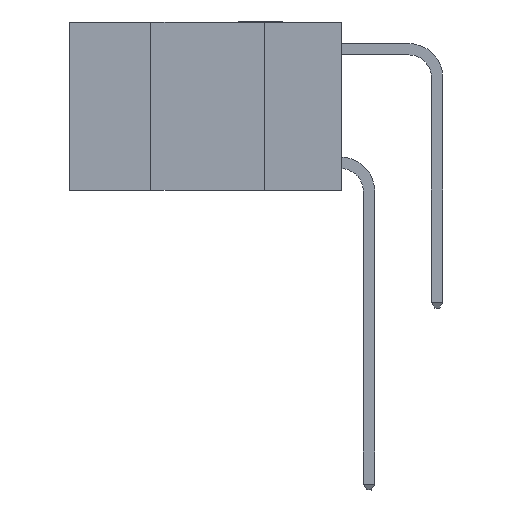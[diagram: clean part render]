
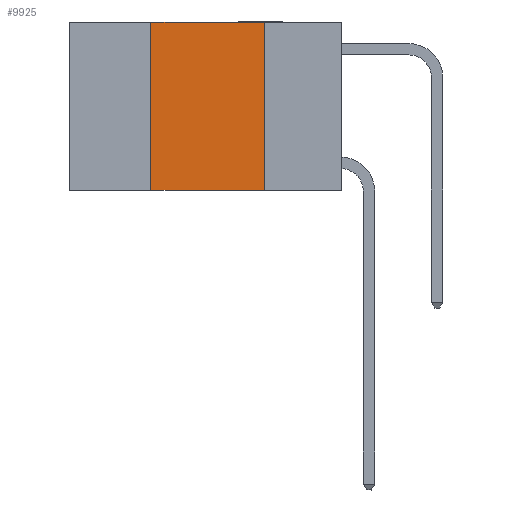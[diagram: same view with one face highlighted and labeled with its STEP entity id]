
A CAD part, left-side view. The second image highlights one B-rep face of the part: STEP entity #9925.
In plain terms, the highlighted planar face has unit normal (-1, 0, 0).
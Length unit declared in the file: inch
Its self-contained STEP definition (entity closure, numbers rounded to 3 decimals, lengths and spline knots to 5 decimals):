
#55 = EDGE_LOOP ( 'NONE', ( #5130, #11378, #8687, #7718 ) ) ;
#657 = AXIS2_PLACEMENT_3D ( 'NONE', #778, #5902, #2843 ) ;
#673 = EDGE_CURVE ( 'NONE', #7932, #5850, #7061, .T. ) ;
#778 = CARTESIAN_POINT ( 'NONE',  ( 0., 0.6, 0. ) ) ;
#857 = DIRECTION ( 'NONE',  ( 0., 0., -1. ) ) ;
#1507 = CARTESIAN_POINT ( 'NONE',  ( 0., 0.42, -0.37 ) ) ;
#1593 = EDGE_CURVE ( 'NONE', #3662, #11846, #10173, .T. ) ;
#2390 = LINE ( 'NONE', #8890, #10620 ) ;
#2830 = EDGE_CURVE ( 'NONE', #11846, #7932, #9328, .T. ) ;
#2843 = DIRECTION ( 'NONE',  ( 0., 0., -1. ) ) ;
#3420 = VECTOR ( 'NONE', #6215, 39.37008 ) ;
#3501 = CARTESIAN_POINT ( 'NONE',  ( 0., 0.17, -0.37 ) ) ;
#3662 = VERTEX_POINT ( 'NONE', #1507 ) ;
#4365 = CARTESIAN_POINT ( 'NONE',  ( 0., 0.6, 0. ) ) ;
#4550 = CARTESIAN_POINT ( 'NONE',  ( 0., 0.42, 0. ) ) ;
#5130 = ORIENTED_EDGE ( 'NONE', *, *, #673, .F. ) ;
#5850 = VERTEX_POINT ( 'NONE', #3501 ) ;
#5902 = DIRECTION ( 'NONE',  ( 1., 0., 0. ) ) ;
#6038 = DIRECTION ( 'NONE',  ( 0., 0., 1. ) ) ;
#6215 = DIRECTION ( 'NONE',  ( 0., -1., 0. ) ) ;
#7061 = LINE ( 'NONE', #8908, #9353 ) ;
#7544 = FACE_OUTER_BOUND ( 'NONE', #55, .T. ) ;
#7718 = ORIENTED_EDGE ( 'NONE', *, *, #11146, .T. ) ;
#7932 = VERTEX_POINT ( 'NONE', #11216 ) ;
#8687 = ORIENTED_EDGE ( 'NONE', *, *, #1593, .F. ) ;
#8810 = CARTESIAN_POINT ( 'NONE',  ( 0., 0.42, 0. ) ) ;
#8890 = CARTESIAN_POINT ( 'NONE',  ( 0., 0.6, -0.37 ) ) ;
#8908 = CARTESIAN_POINT ( 'NONE',  ( 0., 0.17, 0. ) ) ;
#9328 = LINE ( 'NONE', #4365, #3420 ) ;
#9353 = VECTOR ( 'NONE', #857, 39.37008 ) ;
#9893 = PLANE ( 'NONE',  #657 ) ;
#9925 = ADVANCED_FACE ( 'NONE', ( #7544 ), #9893, .F. ) ;
#10173 = LINE ( 'NONE', #8810, #12110 ) ;
#10620 = VECTOR ( 'NONE', #11947, 39.37008 ) ;
#11146 = EDGE_CURVE ( 'NONE', #3662, #5850, #2390, .T. ) ;
#11216 = CARTESIAN_POINT ( 'NONE',  ( 0., 0.17, 0. ) ) ;
#11378 = ORIENTED_EDGE ( 'NONE', *, *, #2830, .F. ) ;
#11846 = VERTEX_POINT ( 'NONE', #4550 ) ;
#11947 = DIRECTION ( 'NONE',  ( 0., -1., 0. ) ) ;
#12110 = VECTOR ( 'NONE', #6038, 39.37008 ) ;
